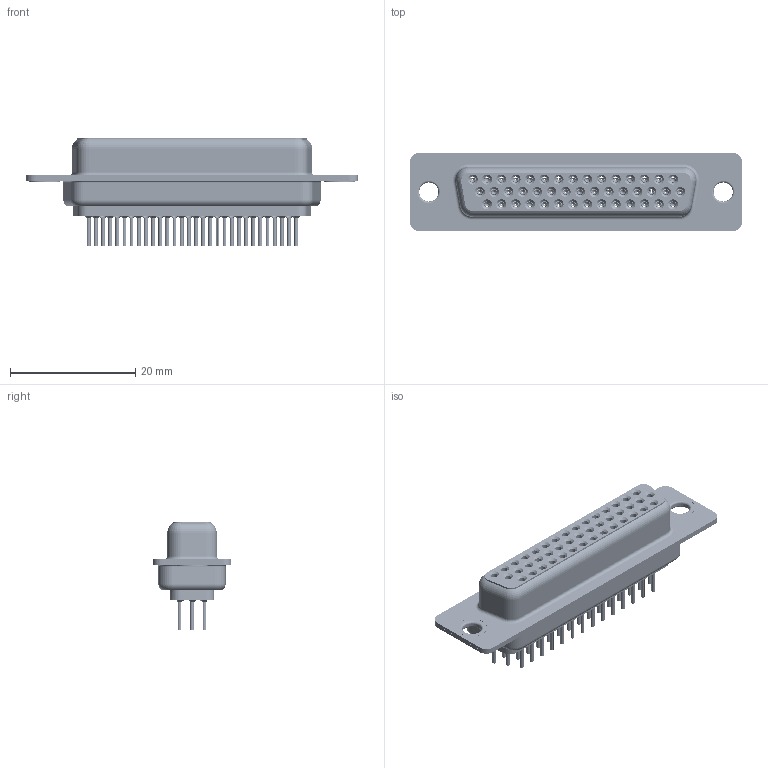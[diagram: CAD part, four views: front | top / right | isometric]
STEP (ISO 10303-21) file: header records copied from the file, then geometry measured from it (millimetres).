
FILE_DESCRIPTION (( 'STEP AP203' ), '1' );
FILE_NAME ('638-044-630-041.STEP', '2020-07-18T23:44:16', ( '' ), ( '' ), 'SwSTEP 2.0', 'SolidWorks 2020', '' );
FILE_SCHEMA (( 'CONFIG_CONTROL_DESIGN' ));
Length unit declared in the file: millimetre
Products named in the file (8): 638-044-630-041; 638 Contact Row 3_30; 638 Shell Rear_44 Contacts; 638 Housing_44 Contacts; 638 Contact Row 1_30; 638 Shell Front_44 Contacts; 638 Contact Row 2_30; 638 Thru Hole Rivet
Assembly tree (49 placements, depth 2):
  638-044-630-041
    638 Housing_44 Contacts
    638 Shell Front_44 Contacts
    638 Shell Rear_44 Contacts
    638 Contact Row 1_30  x15
    638 Contact Row 2_30  x15
    638 Contact Row 3_30  x14
    638 Thru Hole Rivet  x2
Bounding box: 53.04 x 12.6 x 17.3 mm (x, y, z)
Volume: 3185.3 mm3; surface area: 12605.1 mm2
Topology: 49 solids, 49 shells, 5841 faces, 14859 edges, 9215 vertices
Faces by surface type: cylinder 1573, plane 1431, torus 1209, bspline 880, cone 748
Entity records: 38075 total; most frequent: CARTESIAN_POINT 9284, DIRECTION 5985, ORIENTED_EDGE 5336, EDGE_CURVE 2668, AXIS2_PLACEMENT_3D 2526, VERTEX_POINT 1682, CIRCLE 1393, EDGE_LOOP 1384
